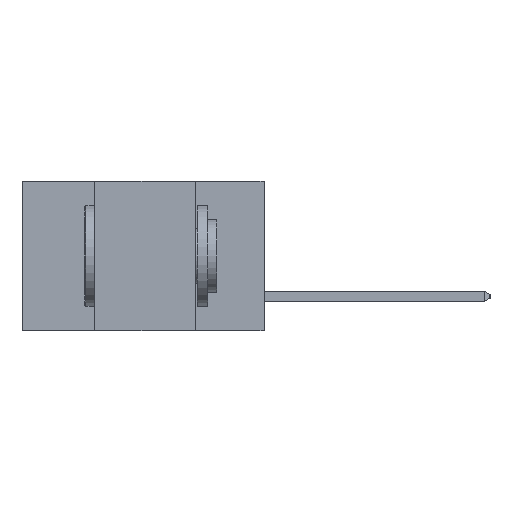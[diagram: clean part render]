
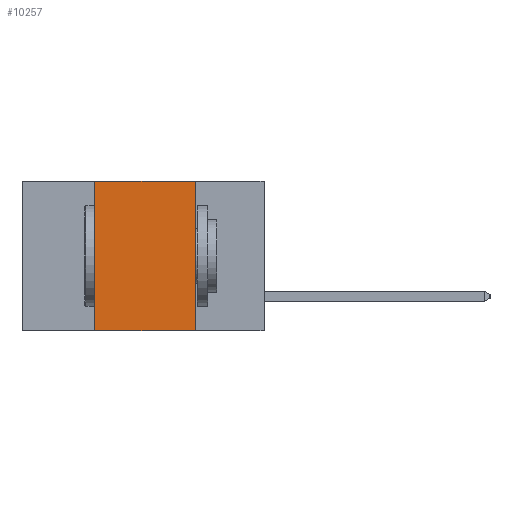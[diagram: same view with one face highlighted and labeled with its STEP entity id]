
A CAD part, left-side view. The second image highlights one B-rep face of the part: STEP entity #10257.
In plain terms, the highlighted planar face has unit normal (-1, 0, 0).
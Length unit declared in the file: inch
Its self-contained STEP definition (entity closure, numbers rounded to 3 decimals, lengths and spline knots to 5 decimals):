
#937 = CARTESIAN_POINT ( 'NONE',  ( 0., 0.6, 0. ) ) ;
#1342 = VECTOR ( 'NONE', #7448, 39.37008 ) ;
#1368 = FACE_OUTER_BOUND ( 'NONE', #3813, .T. ) ;
#2153 = VERTEX_POINT ( 'NONE', #4922 ) ;
#3109 = VECTOR ( 'NONE', #14055, 39.37008 ) ;
#3813 = EDGE_LOOP ( 'NONE', ( #6119, #6636, #7846, #5179 ) ) ;
#3858 = VERTEX_POINT ( 'NONE', #7176 ) ;
#4624 = PLANE ( 'NONE',  #14914 ) ;
#4922 = CARTESIAN_POINT ( 'NONE',  ( 0., 0.17, 0. ) ) ;
#5147 = LINE ( 'NONE', #10960, #8091 ) ;
#5179 = ORIENTED_EDGE ( 'NONE', *, *, #6543, .T. ) ;
#5452 = CARTESIAN_POINT ( 'NONE',  ( 0., 0.6, 0. ) ) ;
#5643 = CARTESIAN_POINT ( 'NONE',  ( 0., 0.17, -0.37 ) ) ;
#5887 = DIRECTION ( 'NONE',  ( 0., 0., -1. ) ) ;
#6119 = ORIENTED_EDGE ( 'NONE', *, *, #6956, .F. ) ;
#6543 = EDGE_CURVE ( 'NONE', #8478, #3858, #5147, .T. ) ;
#6636 = ORIENTED_EDGE ( 'NONE', *, *, #9485, .F. ) ;
#6949 = VERTEX_POINT ( 'NONE', #9374 ) ;
#6956 = EDGE_CURVE ( 'NONE', #2153, #3858, #12163, .T. ) ;
#7176 = CARTESIAN_POINT ( 'NONE',  ( 0., 0.17, -0.37 ) ) ;
#7448 = DIRECTION ( 'NONE',  ( 0., 0., 1. ) ) ;
#7846 = ORIENTED_EDGE ( 'NONE', *, *, #11132, .F. ) ;
#8091 = VECTOR ( 'NONE', #13134, 39.37008 ) ;
#8478 = VERTEX_POINT ( 'NONE', #8554 ) ;
#8554 = CARTESIAN_POINT ( 'NONE',  ( 0., 0.42, -0.37 ) ) ;
#8876 = VECTOR ( 'NONE', #15367, 39.37008 ) ;
#9374 = CARTESIAN_POINT ( 'NONE',  ( 0., 0.42, 0. ) ) ;
#9485 = EDGE_CURVE ( 'NONE', #6949, #2153, #9742, .T. ) ;
#9742 = LINE ( 'NONE', #5452, #3109 ) ;
#10257 = ADVANCED_FACE ( 'NONE', ( #1368 ), #4624, .F. ) ;
#10960 = CARTESIAN_POINT ( 'NONE',  ( 0., 0.6, -0.37 ) ) ;
#11132 = EDGE_CURVE ( 'NONE', #8478, #6949, #11230, .T. ) ;
#11230 = LINE ( 'NONE', #12380, #1342 ) ;
#12163 = LINE ( 'NONE', #5643, #8876 ) ;
#12380 = CARTESIAN_POINT ( 'NONE',  ( 0., 0.42, -0.37 ) ) ;
#13134 = DIRECTION ( 'NONE',  ( 0., -1., 0. ) ) ;
#13283 = DIRECTION ( 'NONE',  ( 1., 0., 0. ) ) ;
#14055 = DIRECTION ( 'NONE',  ( 0., -1., 0. ) ) ;
#14914 = AXIS2_PLACEMENT_3D ( 'NONE', #937, #13283, #5887 ) ;
#15367 = DIRECTION ( 'NONE',  ( 0., 0., -1. ) ) ;
